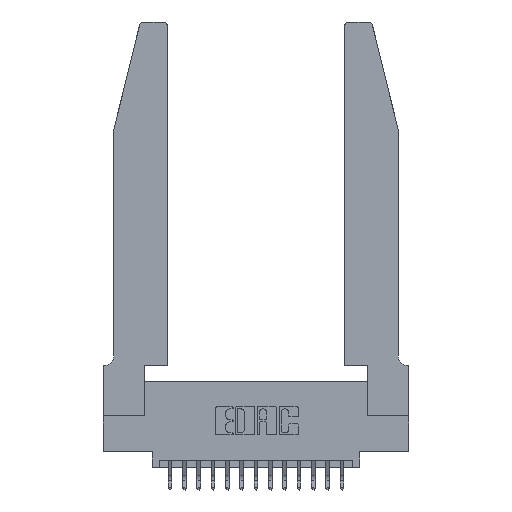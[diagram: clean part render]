
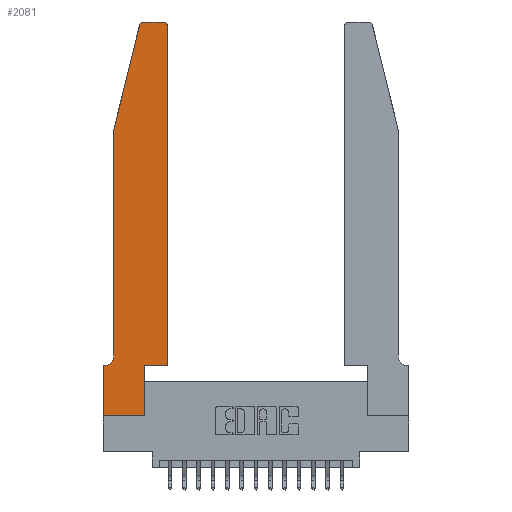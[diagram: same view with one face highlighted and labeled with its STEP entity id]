
A CAD part, top view. The second image highlights one B-rep face of the part: STEP entity #2081.
In plain terms, the highlighted planar face has unit normal (0, 0, 1).
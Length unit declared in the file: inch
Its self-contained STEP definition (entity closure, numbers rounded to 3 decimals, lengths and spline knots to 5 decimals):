
#16 = EDGE_CURVE ( 'NONE', #5879, #1662, #17490, .T. ) ;
#99 = DIRECTION ( 'NONE',  ( 0., -1., 0. ) ) ;
#294 = CARTESIAN_POINT ( 'NONE',  ( 0.0755, 0.42, 0.37 ) ) ;
#326 = VECTOR ( 'NONE', #9457, 39.37008 ) ;
#748 = CARTESIAN_POINT ( 'NONE',  ( 0.2865, 0.35, 0.37 ) ) ;
#947 = DIRECTION ( 'NONE',  ( 0., 0., -1. ) ) ;
#983 = DIRECTION ( 'NONE',  ( 0., 0., 1. ) ) ;
#1392 = CARTESIAN_POINT ( 'NONE',  ( 0.25487, 2.72718, 0.37 ) ) ;
#1467 = AXIS2_PLACEMENT_3D ( 'NONE', #10252, #983, #11688 ) ;
#1555 = CARTESIAN_POINT ( 'NONE',  ( 0., 0., 0.37 ) ) ;
#1577 = VERTEX_POINT ( 'NONE', #6175 ) ;
#1662 = VERTEX_POINT ( 'NONE', #13688 ) ;
#2023 = VECTOR ( 'NONE', #9733, 39.37008 ) ;
#2081 = ADVANCED_FACE ( 'NONE', ( #9659 ), #3623, .T. ) ;
#2308 = EDGE_CURVE ( 'NONE', #7917, #10162, #6857, .T. ) ;
#2356 = DIRECTION ( 'NONE',  ( 1., 0., 0. ) ) ;
#2707 = AXIS2_PLACEMENT_3D ( 'NONE', #12580, #5228, #15461 ) ;
#2715 = EDGE_CURVE ( 'NONE', #6437, #1577, #12518, .T. ) ;
#2759 = VECTOR ( 'NONE', #15481, 39.37008 ) ;
#3050 = CARTESIAN_POINT ( 'NONE',  ( 0.0055, 0.35, 0.37 ) ) ;
#3325 = CIRCLE ( 'NONE', #1467, 0.03 ) ;
#3623 = PLANE ( 'NONE',  #2707 ) ;
#3991 = LINE ( 'NONE', #6164, #15308 ) ;
#4017 = ORIENTED_EDGE ( 'NONE', *, *, #2715, .T. ) ;
#4486 = ORIENTED_EDGE ( 'NONE', *, *, #16355, .T. ) ;
#4989 = EDGE_LOOP ( 'NONE', ( #9708, #14499, #4017, #5803, #16549, #12364, #11349, #18541, #4486, #6862, #18518, #10012 ) ) ;
#5228 = DIRECTION ( 'NONE',  ( 0., 0., 1. ) ) ;
#5803 = ORIENTED_EDGE ( 'NONE', *, *, #6115, .T. ) ;
#5879 = VERTEX_POINT ( 'NONE', #10762 ) ;
#5928 = CARTESIAN_POINT ( 'NONE',  ( 0.4205, 2.72, 0.37 ) ) ;
#6115 = EDGE_CURVE ( 'NONE', #1577, #7917, #10412, .T. ) ;
#6164 = CARTESIAN_POINT ( 'NONE',  ( 0.4505, 0.35, 0.37 ) ) ;
#6175 = CARTESIAN_POINT ( 'NONE',  ( 0.0755, 2., 0.37 ) ) ;
#6437 = VERTEX_POINT ( 'NONE', #1392 ) ;
#6829 = CARTESIAN_POINT ( 'NONE',  ( 0.0755, 2., 0.37 ) ) ;
#6857 = CIRCLE ( 'NONE', #15644, 0.07 ) ;
#6862 = ORIENTED_EDGE ( 'NONE', *, *, #13077, .T. ) ;
#7489 = CARTESIAN_POINT ( 'NONE',  ( 0.4505, 0.35, 0.37 ) ) ;
#7493 = DIRECTION ( 'NONE',  ( 1., 0., 0. ) ) ;
#7636 = LINE ( 'NONE', #17118, #14392 ) ;
#7689 = CARTESIAN_POINT ( 'NONE',  ( 0.4205, 2.75, 0.37 ) ) ;
#7708 = DIRECTION ( 'NONE',  ( 0., 1., 0. ) ) ;
#7917 = VERTEX_POINT ( 'NONE', #294 ) ;
#7963 = EDGE_CURVE ( 'NONE', #10162, #5879, #9762, .T. ) ;
#8321 = CARTESIAN_POINT ( 'NONE',  ( 0.4505, 2.72, 0.37 ) ) ;
#8400 = VECTOR ( 'NONE', #8747, 39.37008 ) ;
#8747 = DIRECTION ( 'NONE',  ( -1., 0., 0. ) ) ;
#8815 = EDGE_CURVE ( 'NONE', #17363, #10377, #3991, .T. ) ;
#9302 = LINE ( 'NONE', #11555, #8400 ) ;
#9457 = DIRECTION ( 'NONE',  ( -0.239, -0.971, 0. ) ) ;
#9659 = FACE_OUTER_BOUND ( 'NONE', #4989, .T. ) ;
#9708 = ORIENTED_EDGE ( 'NONE', *, *, #15091, .T. ) ;
#9733 = DIRECTION ( 'NONE',  ( -1., 0., 0. ) ) ;
#9762 = LINE ( 'NONE', #12584, #2023 ) ;
#10012 = ORIENTED_EDGE ( 'NONE', *, *, #15182, .T. ) ;
#10162 = VERTEX_POINT ( 'NONE', #3050 ) ;
#10216 = CARTESIAN_POINT ( 'NONE',  ( 0.0055, 0.42, 0.37 ) ) ;
#10252 = CARTESIAN_POINT ( 'NONE',  ( 0.284, 2.72, 0.37 ) ) ;
#10377 = VERTEX_POINT ( 'NONE', #8321 ) ;
#10412 = LINE ( 'NONE', #6829, #2759 ) ;
#10514 = EDGE_CURVE ( 'NONE', #1662, #16090, #7636, .T. ) ;
#10721 = LINE ( 'NONE', #10736, #18250 ) ;
#10736 = CARTESIAN_POINT ( 'NONE',  ( 0.4505, 0.35, 0.37 ) ) ;
#10762 = CARTESIAN_POINT ( 'NONE',  ( 0., 0.35, 0.37 ) ) ;
#10865 = CIRCLE ( 'NONE', #15704, 0.03 ) ;
#11115 = CARTESIAN_POINT ( 'NONE',  ( 0.284, 2.75, 0.37 ) ) ;
#11349 = ORIENTED_EDGE ( 'NONE', *, *, #16, .T. ) ;
#11465 = CARTESIAN_POINT ( 'NONE',  ( 0.2865, 0., 0.37 ) ) ;
#11555 = CARTESIAN_POINT ( 'NONE',  ( 0.2605, 2.75, 0.37 ) ) ;
#11654 = DIRECTION ( 'NONE',  ( -1., 0., 0. ) ) ;
#11688 = DIRECTION ( 'NONE',  ( 1., 0., 0. ) ) ;
#12364 = ORIENTED_EDGE ( 'NONE', *, *, #7963, .T. ) ;
#12518 = LINE ( 'NONE', #16560, #326 ) ;
#12580 = CARTESIAN_POINT ( 'NONE',  ( 0., 0.35, 0.37 ) ) ;
#12584 = CARTESIAN_POINT ( 'NONE',  ( 0.0755, 0.35, 0.37 ) ) ;
#12747 = VERTEX_POINT ( 'NONE', #748 ) ;
#13077 = EDGE_CURVE ( 'NONE', #12747, #17363, #10721, .T. ) ;
#13431 = CARTESIAN_POINT ( 'NONE',  ( 0.2865, 0.35, 0.37 ) ) ;
#13688 = CARTESIAN_POINT ( 'NONE',  ( 0., 0., 0.37 ) ) ;
#13700 = VECTOR ( 'NONE', #99, 39.37008 ) ;
#13934 = VECTOR ( 'NONE', #7708, 39.37008 ) ;
#14392 = VECTOR ( 'NONE', #2356, 39.37008 ) ;
#14499 = ORIENTED_EDGE ( 'NONE', *, *, #19004, .T. ) ;
#14877 = DIRECTION ( 'NONE',  ( 0., 1., 0. ) ) ;
#15027 = DIRECTION ( 'NONE',  ( 1., 0., 0. ) ) ;
#15091 = EDGE_CURVE ( 'NONE', #19146, #17033, #9302, .T. ) ;
#15182 = EDGE_CURVE ( 'NONE', #10377, #19146, #10865, .T. ) ;
#15308 = VECTOR ( 'NONE', #14877, 39.37008 ) ;
#15461 = DIRECTION ( 'NONE',  ( 1., 0., 0. ) ) ;
#15481 = DIRECTION ( 'NONE',  ( 0., -1., 0. ) ) ;
#15644 = AXIS2_PLACEMENT_3D ( 'NONE', #10216, #947, #11654 ) ;
#15704 = AXIS2_PLACEMENT_3D ( 'NONE', #5928, #16089, #7493 ) ;
#16089 = DIRECTION ( 'NONE',  ( 0., 0., 1. ) ) ;
#16090 = VERTEX_POINT ( 'NONE', #11465 ) ;
#16355 = EDGE_CURVE ( 'NONE', #16090, #12747, #17705, .T. ) ;
#16549 = ORIENTED_EDGE ( 'NONE', *, *, #2308, .T. ) ;
#16560 = CARTESIAN_POINT ( 'NONE',  ( 0.0755, 2., 0.37 ) ) ;
#17033 = VERTEX_POINT ( 'NONE', #11115 ) ;
#17118 = CARTESIAN_POINT ( 'NONE',  ( 0., 0., 0.37 ) ) ;
#17363 = VERTEX_POINT ( 'NONE', #7489 ) ;
#17490 = LINE ( 'NONE', #1555, #13700 ) ;
#17705 = LINE ( 'NONE', #13431, #13934 ) ;
#18250 = VECTOR ( 'NONE', #15027, 39.37008 ) ;
#18518 = ORIENTED_EDGE ( 'NONE', *, *, #8815, .T. ) ;
#18541 = ORIENTED_EDGE ( 'NONE', *, *, #10514, .T. ) ;
#19004 = EDGE_CURVE ( 'NONE', #17033, #6437, #3325, .T. ) ;
#19146 = VERTEX_POINT ( 'NONE', #7689 ) ;
